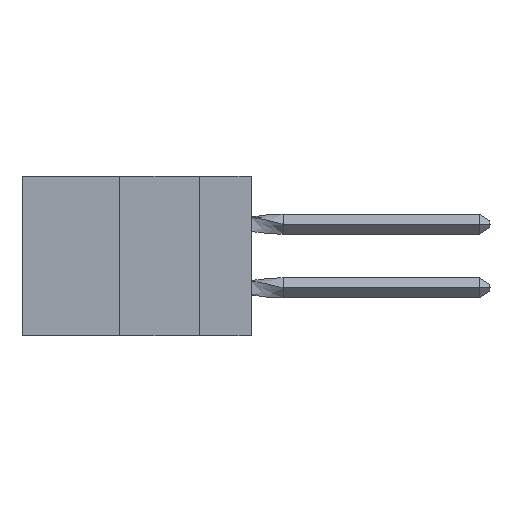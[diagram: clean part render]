
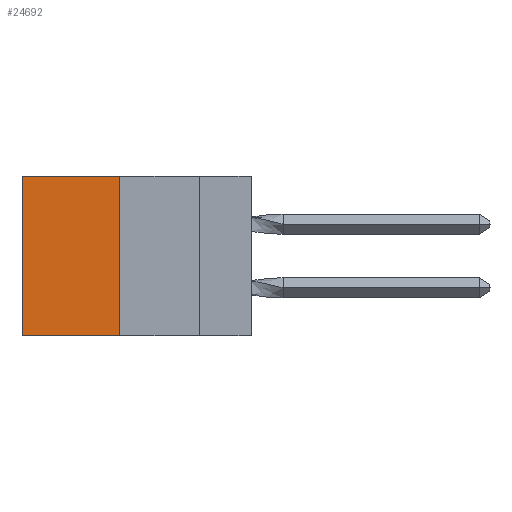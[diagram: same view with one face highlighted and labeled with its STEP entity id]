
A CAD part, left-side view. The second image highlights one B-rep face of the part: STEP entity #24692.
In plain terms, the highlighted planar face has unit normal (-1, 0, 0).
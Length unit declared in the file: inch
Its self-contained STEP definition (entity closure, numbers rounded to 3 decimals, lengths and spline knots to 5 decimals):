
#150 = ORIENTED_EDGE ( 'NONE', *, *, #23752, .T. ) ;
#245 = EDGE_CURVE ( 'NONE', #14484, #15393, #13386, .T. ) ;
#454 = CARTESIAN_POINT ( 'NONE',  ( 0.305, 0.413, -0.5 ) ) ;
#5285 = VECTOR ( 'NONE', #16350, 39.37008 ) ;
#5779 = AXIS2_PLACEMENT_3D ( 'NONE', #9411, #30996, #28591 ) ;
#6667 = VECTOR ( 'NONE', #21971, 39.37008 ) ;
#9411 = CARTESIAN_POINT ( 'NONE',  ( 0.305, 0.413, -0.5 ) ) ;
#11289 = CARTESIAN_POINT ( 'NONE',  ( 0.305, 0.413, 0. ) ) ;
#11569 = VERTEX_POINT ( 'NONE', #19154 ) ;
#13386 = LINE ( 'NONE', #454, #6667 ) ;
#14049 = CARTESIAN_POINT ( 'NONE',  ( 0.305, 0.72, -0.5 ) ) ;
#14484 = VERTEX_POINT ( 'NONE', #19657 ) ;
#14943 = EDGE_CURVE ( 'NONE', #30667, #11569, #20639, .T. ) ;
#15393 = VERTEX_POINT ( 'NONE', #16930 ) ;
#15640 = EDGE_CURVE ( 'NONE', #30667, #14484, #19873, .T. ) ;
#16340 = FACE_OUTER_BOUND ( 'NONE', #19296, .T. ) ;
#16350 = DIRECTION ( 'NONE',  ( 0., 0., -1. ) ) ;
#16851 = CARTESIAN_POINT ( 'NONE',  ( 0.305, 0.413, 0. ) ) ;
#16930 = CARTESIAN_POINT ( 'NONE',  ( 0.305, 0.72, -0.5 ) ) ;
#19154 = CARTESIAN_POINT ( 'NONE',  ( 0.305, 0.72, 0. ) ) ;
#19296 = EDGE_LOOP ( 'NONE', ( #150, #24368, #23008, #30050 ) ) ;
#19657 = CARTESIAN_POINT ( 'NONE',  ( 0.305, 0.413, -0.5 ) ) ;
#19873 = LINE ( 'NONE', #27970, #5285 ) ;
#20639 = LINE ( 'NONE', #11289, #22493 ) ;
#20962 = DIRECTION ( 'NONE',  ( 0., 1., 0. ) ) ;
#21606 = LINE ( 'NONE', #14049, #23837 ) ;
#21971 = DIRECTION ( 'NONE',  ( 0., 1., 0. ) ) ;
#22493 = VECTOR ( 'NONE', #20962, 39.37008 ) ;
#23008 = ORIENTED_EDGE ( 'NONE', *, *, #15640, .F. ) ;
#23574 = DIRECTION ( 'NONE',  ( 0., 0., -1. ) ) ;
#23752 = EDGE_CURVE ( 'NONE', #11569, #15393, #21606, .T. ) ;
#23837 = VECTOR ( 'NONE', #23574, 39.37008 ) ;
#24368 = ORIENTED_EDGE ( 'NONE', *, *, #245, .F. ) ;
#24692 = ADVANCED_FACE ( 'NONE', ( #16340 ), #25735, .F. ) ;
#25735 = PLANE ( 'NONE',  #5779 ) ;
#27970 = CARTESIAN_POINT ( 'NONE',  ( 0.305, 0.413, -0.5 ) ) ;
#28591 = DIRECTION ( 'NONE',  ( 0., 0., -1. ) ) ;
#30050 = ORIENTED_EDGE ( 'NONE', *, *, #14943, .T. ) ;
#30667 = VERTEX_POINT ( 'NONE', #16851 ) ;
#30996 = DIRECTION ( 'NONE',  ( 1., 0., 0. ) ) ;
